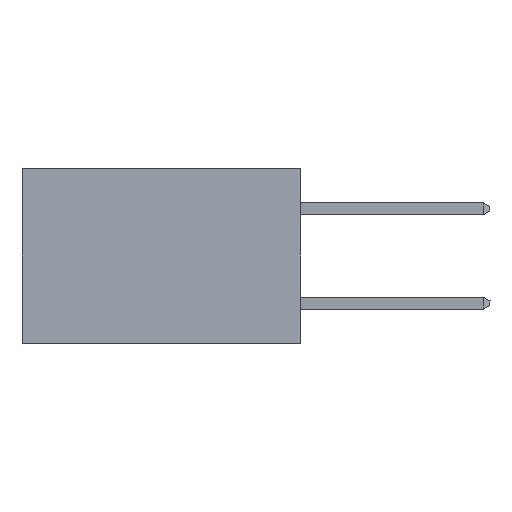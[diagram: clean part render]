
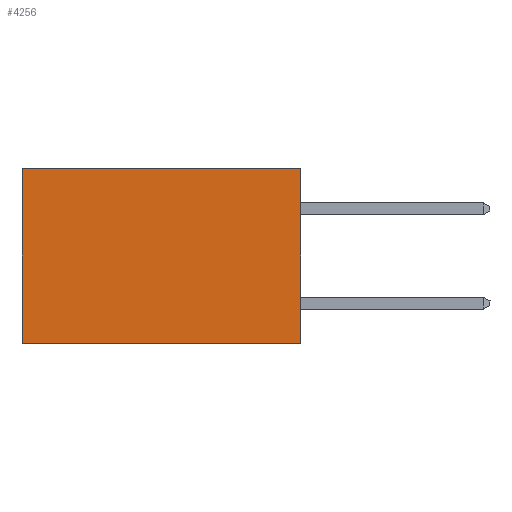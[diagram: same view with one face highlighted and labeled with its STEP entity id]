
A CAD part, left-side view. The second image highlights one B-rep face of the part: STEP entity #4256.
In plain terms, the highlighted planar face has unit normal (-1, 0, 0).
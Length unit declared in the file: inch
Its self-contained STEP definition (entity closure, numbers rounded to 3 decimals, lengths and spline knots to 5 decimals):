
#250 = CARTESIAN_POINT ( 'NONE',  ( 0.277, 0., 0. ) ) ;
#327 = AXIS2_PLACEMENT_3D ( 'NONE', #5693, #5616, #5591 ) ;
#536 = VERTEX_POINT ( 'NONE', #3687 ) ;
#594 = VECTOR ( 'NONE', #3143, 39.37008 ) ;
#619 = ORIENTED_EDGE ( 'NONE', *, *, #1075, .T. ) ;
#625 = ORIENTED_EDGE ( 'NONE', *, *, #1768, .F. ) ;
#658 = ORIENTED_EDGE ( 'NONE', *, *, #1777, .F. ) ;
#684 = ORIENTED_EDGE ( 'NONE', *, *, #930, .T. ) ;
#930 = EDGE_CURVE ( 'NONE', #3288, #536, #6601, .T. ) ;
#1075 = EDGE_CURVE ( 'NONE', #536, #7144, #5204, .T. ) ;
#1112 = FACE_OUTER_BOUND ( 'NONE', #2617, .T. ) ;
#1768 = EDGE_CURVE ( 'NONE', #1860, #7144, #7094, .T. ) ;
#1777 = EDGE_CURVE ( 'NONE', #3288, #1860, #4097, .T. ) ;
#1860 = VERTEX_POINT ( 'NONE', #4339 ) ;
#2305 = CARTESIAN_POINT ( 'NONE',  ( 0.277, 0., 0. ) ) ;
#2617 = EDGE_LOOP ( 'NONE', ( #619, #625, #658, #684 ) ) ;
#2658 = VECTOR ( 'NONE', #6851, 39.37008 ) ;
#3143 = DIRECTION ( 'NONE',  ( 0., 0., -1. ) ) ;
#3288 = VERTEX_POINT ( 'NONE', #2305 ) ;
#3348 = CARTESIAN_POINT ( 'NONE',  ( 0.277, 0., -0.37 ) ) ;
#3687 = CARTESIAN_POINT ( 'NONE',  ( 0.277, 0.59, 0. ) ) ;
#4097 = LINE ( 'NONE', #3348, #594 ) ;
#4256 = ADVANCED_FACE ( 'NONE', ( #1112 ), #5635, .F. ) ;
#4339 = CARTESIAN_POINT ( 'NONE',  ( 0.277, 0., -0.37 ) ) ;
#4504 = CARTESIAN_POINT ( 'NONE',  ( 0.277, 0.59, -0.37 ) ) ;
#4589 = CARTESIAN_POINT ( 'NONE',  ( 0.277, 0.59, -0.37 ) ) ;
#5005 = VECTOR ( 'NONE', #5604, 39.37008 ) ;
#5204 = LINE ( 'NONE', #4504, #5005 ) ;
#5591 = DIRECTION ( 'NONE',  ( 0., 0., -1. ) ) ;
#5604 = DIRECTION ( 'NONE',  ( 0., 0., -1. ) ) ;
#5616 = DIRECTION ( 'NONE',  ( 1., 0., 0. ) ) ;
#5635 = PLANE ( 'NONE',  #327 ) ;
#5693 = CARTESIAN_POINT ( 'NONE',  ( 0.277, 0., -0.37 ) ) ;
#6308 = CARTESIAN_POINT ( 'NONE',  ( 0.277, 0., -0.37 ) ) ;
#6465 = VECTOR ( 'NONE', #6481, 39.37008 ) ;
#6481 = DIRECTION ( 'NONE',  ( 0., 1., 0. ) ) ;
#6601 = LINE ( 'NONE', #250, #6465 ) ;
#6851 = DIRECTION ( 'NONE',  ( 0., 1., 0. ) ) ;
#7094 = LINE ( 'NONE', #6308, #2658 ) ;
#7144 = VERTEX_POINT ( 'NONE', #4589 ) ;
